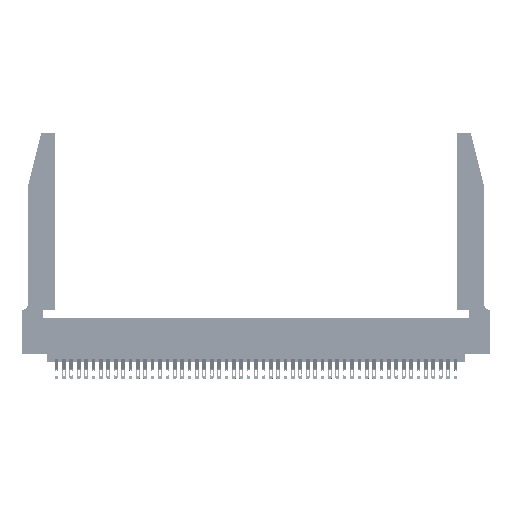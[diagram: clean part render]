
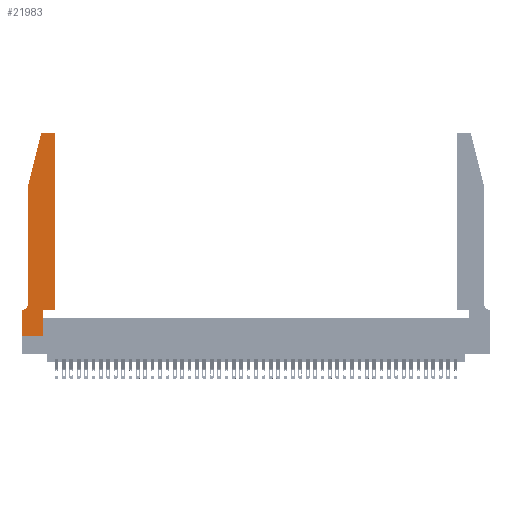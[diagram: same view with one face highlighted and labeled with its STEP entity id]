
A CAD part, top view. The second image highlights one B-rep face of the part: STEP entity #21983.
In plain terms, the highlighted planar face has unit normal (0, 0, 1).
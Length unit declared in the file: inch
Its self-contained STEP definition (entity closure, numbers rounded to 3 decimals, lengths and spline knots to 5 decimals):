
#297 = ORIENTED_EDGE ( 'NONE', *, *, #14437, .T. ) ;
#787 = DIRECTION ( 'NONE',  ( 0., 0., 1. ) ) ;
#804 = CARTESIAN_POINT ( 'NONE',  ( 0., 0., 0.37 ) ) ;
#812 = VECTOR ( 'NONE', #31074, 39.37008 ) ;
#967 = VERTEX_POINT ( 'NONE', #35742 ) ;
#1036 = LINE ( 'NONE', #1707, #41205 ) ;
#1040 = CARTESIAN_POINT ( 'NONE',  ( 0.4505, 0.35, 0.37 ) ) ;
#1230 = EDGE_CURVE ( 'NONE', #13538, #41418, #30646, .T. ) ;
#1707 = CARTESIAN_POINT ( 'NONE',  ( 0., 0., 0.37 ) ) ;
#2516 = CARTESIAN_POINT ( 'NONE',  ( 0.4205, 2.75, 0.37 ) ) ;
#2526 = CARTESIAN_POINT ( 'NONE',  ( 0.0055, 0.35, 0.37 ) ) ;
#2878 = CARTESIAN_POINT ( 'NONE',  ( 0.2865, 0.35, 0.37 ) ) ;
#2995 = VERTEX_POINT ( 'NONE', #3577 ) ;
#3347 = LINE ( 'NONE', #38649, #42802 ) ;
#3577 = CARTESIAN_POINT ( 'NONE',  ( 0., 0.35, 0.37 ) ) ;
#3773 = VECTOR ( 'NONE', #11885, 39.37008 ) ;
#3875 = EDGE_CURVE ( 'NONE', #33944, #34549, #23616, .T. ) ;
#4345 = VECTOR ( 'NONE', #15520, 39.37008 ) ;
#4890 = VERTEX_POINT ( 'NONE', #36512 ) ;
#4952 = CARTESIAN_POINT ( 'NONE',  ( 0., 0., 0.37 ) ) ;
#5074 = DIRECTION ( 'NONE',  ( 0., 1., 0. ) ) ;
#5262 = CARTESIAN_POINT ( 'NONE',  ( 0.4205, 2.72, 0.37 ) ) ;
#5494 = EDGE_CURVE ( 'NONE', #28601, #33944, #13920, .T. ) ;
#6676 = ORIENTED_EDGE ( 'NONE', *, *, #13406, .T. ) ;
#8001 = EDGE_CURVE ( 'NONE', #35756, #13538, #38285, .T. ) ;
#8213 = EDGE_CURVE ( 'NONE', #2995, #35756, #1036, .T. ) ;
#8677 = VECTOR ( 'NONE', #5074, 39.37008 ) ;
#8989 = CARTESIAN_POINT ( 'NONE',  ( 0.284, 2.75, 0.37 ) ) ;
#9958 = ORIENTED_EDGE ( 'NONE', *, *, #8001, .T. ) ;
#10278 = ORIENTED_EDGE ( 'NONE', *, *, #3875, .T. ) ;
#11150 = CARTESIAN_POINT ( 'NONE',  ( 0., 0.35, 0.37 ) ) ;
#11197 = ORIENTED_EDGE ( 'NONE', *, *, #11847, .T. ) ;
#11330 = DIRECTION ( 'NONE',  ( 1., 0., 0. ) ) ;
#11637 = AXIS2_PLACEMENT_3D ( 'NONE', #45308, #30490, #30639 ) ;
#11847 = EDGE_CURVE ( 'NONE', #43876, #967, #42477, .T. ) ;
#11885 = DIRECTION ( 'NONE',  ( 0., -1., 0. ) ) ;
#13178 = CARTESIAN_POINT ( 'NONE',  ( 0.4505, 0.35, 0.37 ) ) ;
#13406 = EDGE_CURVE ( 'NONE', #41418, #28601, #3347, .T. ) ;
#13538 = VERTEX_POINT ( 'NONE', #27008 ) ;
#13920 = LINE ( 'NONE', #1040, #4345 ) ;
#14437 = EDGE_CURVE ( 'NONE', #967, #4890, #31380, .T. ) ;
#15520 = DIRECTION ( 'NONE',  ( 0., 1., 0. ) ) ;
#15929 = CARTESIAN_POINT ( 'NONE',  ( 0.25487, 2.72718, 0.37 ) ) ;
#15958 = EDGE_CURVE ( 'NONE', #34549, #25861, #19973, .T. ) ;
#17537 = LINE ( 'NONE', #45379, #27669 ) ;
#18853 = PLANE ( 'NONE',  #22508 ) ;
#19403 = CARTESIAN_POINT ( 'NONE',  ( 0.2865, 0.35, 0.37 ) ) ;
#19973 = LINE ( 'NONE', #38045, #812 ) ;
#20709 = ORIENTED_EDGE ( 'NONE', *, *, #15958, .T. ) ;
#20815 = EDGE_CURVE ( 'NONE', #4890, #30165, #30641, .T. ) ;
#21343 = DIRECTION ( 'NONE',  ( 1., 0., 0. ) ) ;
#21983 = ADVANCED_FACE ( 'NONE', ( #37915 ), #18853, .T. ) ;
#22508 = AXIS2_PLACEMENT_3D ( 'NONE', #11150, #787, #33373 ) ;
#22679 = DIRECTION ( 'NONE',  ( -0.239, -0.971, 0. ) ) ;
#23616 = CIRCLE ( 'NONE', #31792, 0.03 ) ;
#23856 = ORIENTED_EDGE ( 'NONE', *, *, #1230, .T. ) ;
#24155 = VECTOR ( 'NONE', #45568, 39.37008 ) ;
#24239 = CARTESIAN_POINT ( 'NONE',  ( 0.4505, 2.72, 0.37 ) ) ;
#24849 = EDGE_CURVE ( 'NONE', #25861, #43876, #35957, .T. ) ;
#25269 = DIRECTION ( 'NONE',  ( 0., 0., 1. ) ) ;
#25861 = VERTEX_POINT ( 'NONE', #8989 ) ;
#26998 = DIRECTION ( 'NONE',  ( 1., 0., 0. ) ) ;
#27008 = CARTESIAN_POINT ( 'NONE',  ( 0.2865, 0., 0.37 ) ) ;
#27669 = VECTOR ( 'NONE', #45850, 39.37008 ) ;
#28601 = VERTEX_POINT ( 'NONE', #13178 ) ;
#28729 = ORIENTED_EDGE ( 'NONE', *, *, #20815, .T. ) ;
#30165 = VERTEX_POINT ( 'NONE', #2526 ) ;
#30402 = CARTESIAN_POINT ( 'NONE',  ( 0.0755, 2., 0.37 ) ) ;
#30490 = DIRECTION ( 'NONE',  ( 0., 0., -1. ) ) ;
#30639 = DIRECTION ( 'NONE',  ( -1., 0., 0. ) ) ;
#30641 = CIRCLE ( 'NONE', #11637, 0.07 ) ;
#30646 = LINE ( 'NONE', #19403, #8677 ) ;
#31074 = DIRECTION ( 'NONE',  ( -1., 0., 0. ) ) ;
#31097 = DIRECTION ( 'NONE',  ( 0., 0., 1. ) ) ;
#31285 = ORIENTED_EDGE ( 'NONE', *, *, #24849, .T. ) ;
#31380 = LINE ( 'NONE', #39925, #3773 ) ;
#31792 = AXIS2_PLACEMENT_3D ( 'NONE', #5262, #31097, #26998 ) ;
#32822 = VECTOR ( 'NONE', #22679, 39.37008 ) ;
#33373 = DIRECTION ( 'NONE',  ( 1., 0., 0. ) ) ;
#33622 = ORIENTED_EDGE ( 'NONE', *, *, #8213, .T. ) ;
#33944 = VERTEX_POINT ( 'NONE', #24239 ) ;
#34549 = VERTEX_POINT ( 'NONE', #2516 ) ;
#35742 = CARTESIAN_POINT ( 'NONE',  ( 0.0755, 2., 0.37 ) ) ;
#35756 = VERTEX_POINT ( 'NONE', #4952 ) ;
#35957 = CIRCLE ( 'NONE', #40439, 0.03 ) ;
#36512 = CARTESIAN_POINT ( 'NONE',  ( 0.0755, 0.42, 0.37 ) ) ;
#36943 = ORIENTED_EDGE ( 'NONE', *, *, #38967, .T. ) ;
#37915 = FACE_OUTER_BOUND ( 'NONE', #43145, .T. ) ;
#38045 = CARTESIAN_POINT ( 'NONE',  ( 0.2605, 2.75, 0.37 ) ) ;
#38285 = LINE ( 'NONE', #804, #24155 ) ;
#38649 = CARTESIAN_POINT ( 'NONE',  ( 0.4505, 0.35, 0.37 ) ) ;
#38967 = EDGE_CURVE ( 'NONE', #30165, #2995, #17537, .T. ) ;
#39925 = CARTESIAN_POINT ( 'NONE',  ( 0.0755, 2., 0.37 ) ) ;
#40439 = AXIS2_PLACEMENT_3D ( 'NONE', #46580, #25269, #21343 ) ;
#41205 = VECTOR ( 'NONE', #41403, 39.37008 ) ;
#41403 = DIRECTION ( 'NONE',  ( 0., -1., 0. ) ) ;
#41418 = VERTEX_POINT ( 'NONE', #2878 ) ;
#42477 = LINE ( 'NONE', #30402, #32822 ) ;
#42802 = VECTOR ( 'NONE', #11330, 39.37008 ) ;
#43145 = EDGE_LOOP ( 'NONE', ( #20709, #31285, #11197, #297, #28729, #36943, #33622, #9958, #23856, #6676, #45959, #10278 ) ) ;
#43876 = VERTEX_POINT ( 'NONE', #15929 ) ;
#45308 = CARTESIAN_POINT ( 'NONE',  ( 0.0055, 0.42, 0.37 ) ) ;
#45379 = CARTESIAN_POINT ( 'NONE',  ( 0.0755, 0.35, 0.37 ) ) ;
#45568 = DIRECTION ( 'NONE',  ( 1., 0., 0. ) ) ;
#45850 = DIRECTION ( 'NONE',  ( -1., 0., 0. ) ) ;
#45959 = ORIENTED_EDGE ( 'NONE', *, *, #5494, .T. ) ;
#46580 = CARTESIAN_POINT ( 'NONE',  ( 0.284, 2.72, 0.37 ) ) ;
